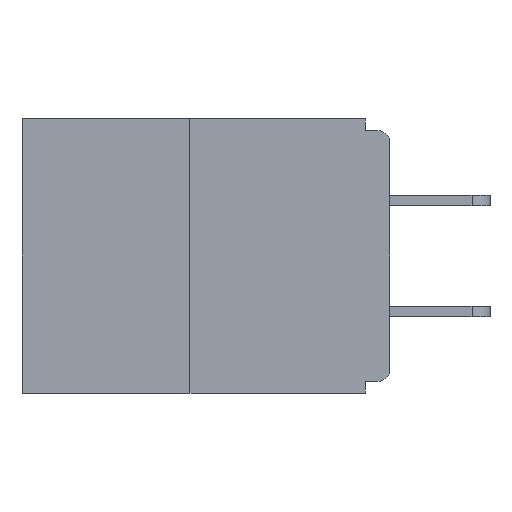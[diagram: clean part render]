
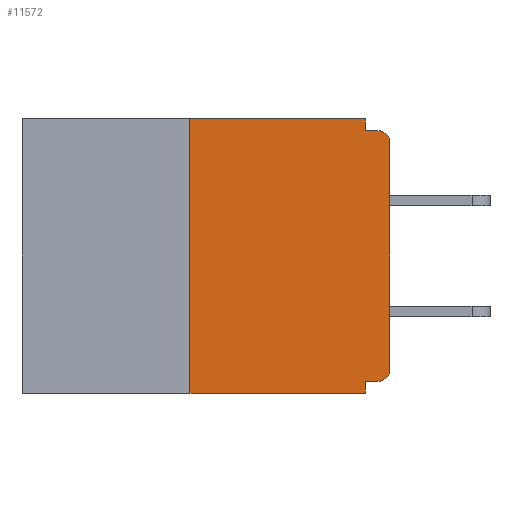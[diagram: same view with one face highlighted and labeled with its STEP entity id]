
A CAD part, left-side view. The second image highlights one B-rep face of the part: STEP entity #11572.
In plain terms, the highlighted planar face has unit normal (-1, 0, 0).
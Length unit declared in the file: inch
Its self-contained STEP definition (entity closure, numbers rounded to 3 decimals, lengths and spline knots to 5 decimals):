
#219 = DIRECTION ( 'NONE',  ( 0., -1., 0. ) ) ;
#304 = EDGE_CURVE ( 'NONE', #12619, #564, #17571, .T. ) ;
#513 = ORIENTED_EDGE ( 'NONE', *, *, #15176, .F. ) ;
#564 = VERTEX_POINT ( 'NONE', #8336 ) ;
#835 = DIRECTION ( 'NONE',  ( -1., 0., 0. ) ) ;
#873 = CARTESIAN_POINT ( 'NONE',  ( 0., 0.015, -0.313 ) ) ;
#932 = DIRECTION ( 'NONE',  ( 0., 1., 0. ) ) ;
#1701 = CARTESIAN_POINT ( 'NONE',  ( 0., 0.031, 0. ) ) ;
#1729 = EDGE_CURVE ( 'NONE', #12619, #13529, #4826, .T. ) ;
#1971 = ORIENTED_EDGE ( 'NONE', *, *, #9385, .F. ) ;
#2125 = ORIENTED_EDGE ( 'NONE', *, *, #1729, .F. ) ;
#2174 = CARTESIAN_POINT ( 'NONE',  ( 0., 0.015, -0.03 ) ) ;
#2514 = EDGE_CURVE ( 'NONE', #12037, #9377, #8472, .T. ) ;
#2839 = VECTOR ( 'NONE', #4182, 39.37008 ) ;
#2876 = DIRECTION ( 'NONE',  ( 0., 0., -1. ) ) ;
#3122 = CARTESIAN_POINT ( 'NONE',  ( 0., 0.25, -0.343 ) ) ;
#3673 = ORIENTED_EDGE ( 'NONE', *, *, #17015, .T. ) ;
#3957 = VERTEX_POINT ( 'NONE', #3960 ) ;
#3960 = CARTESIAN_POINT ( 'NONE',  ( 0., 0., -0.03 ) ) ;
#4057 = CARTESIAN_POINT ( 'NONE',  ( 0., 0., 0. ) ) ;
#4182 = DIRECTION ( 'NONE',  ( 0., 0., 1. ) ) ;
#4380 = CARTESIAN_POINT ( 'NONE',  ( 0., 0.031, 0. ) ) ;
#4469 = ORIENTED_EDGE ( 'NONE', *, *, #5813, .F. ) ;
#4684 = ORIENTED_EDGE ( 'NONE', *, *, #2514, .F. ) ;
#4826 = LINE ( 'NONE', #6350, #11333 ) ;
#4979 = DIRECTION ( 'NONE',  ( 1., 0., 0. ) ) ;
#5468 = EDGE_CURVE ( 'NONE', #15251, #14833, #17730, .T. ) ;
#5727 = CARTESIAN_POINT ( 'NONE',  ( 0., 0.031, -0.015 ) ) ;
#5813 = EDGE_CURVE ( 'NONE', #13546, #564, #14965, .T. ) ;
#6093 = ORIENTED_EDGE ( 'NONE', *, *, #8663, .T. ) ;
#6254 = CARTESIAN_POINT ( 'NONE',  ( 0., 0., -0.015 ) ) ;
#6350 = CARTESIAN_POINT ( 'NONE',  ( 0., 0.25, 0. ) ) ;
#6360 = DIRECTION ( 'NONE',  ( 0., 0., -1. ) ) ;
#6596 = EDGE_LOOP ( 'NONE', ( #1971, #2125, #8793, #4469, #10486, #12529, #6093, #3673, #513, #4684 ) ) ;
#6995 = CARTESIAN_POINT ( 'NONE',  ( 0., 0.46, 0. ) ) ;
#7605 = CARTESIAN_POINT ( 'NONE',  ( 0., 0.25, 0. ) ) ;
#7823 = VECTOR ( 'NONE', #2876, 39.37008 ) ;
#7994 = LINE ( 'NONE', #4057, #2839 ) ;
#8002 = CARTESIAN_POINT ( 'NONE',  ( 0., 0.015, -0.015 ) ) ;
#8170 = VECTOR ( 'NONE', #219, 39.37008 ) ;
#8336 = CARTESIAN_POINT ( 'NONE',  ( 0., 0.031, -0.343 ) ) ;
#8472 = LINE ( 'NONE', #4380, #7823 ) ;
#8663 = EDGE_CURVE ( 'NONE', #14833, #3957, #7994, .T. ) ;
#8750 = CARTESIAN_POINT ( 'NONE',  ( 0., 0.46, -0.343 ) ) ;
#8793 = ORIENTED_EDGE ( 'NONE', *, *, #304, .T. ) ;
#9377 = VERTEX_POINT ( 'NONE', #5727 ) ;
#9385 = EDGE_CURVE ( 'NONE', #13529, #12037, #9483, .T. ) ;
#9483 = LINE ( 'NONE', #6995, #8170 ) ;
#9524 = CARTESIAN_POINT ( 'NONE',  ( 0., 0.015, -0.328 ) ) ;
#9771 = VECTOR ( 'NONE', #932, 39.37008 ) ;
#10486 = ORIENTED_EDGE ( 'NONE', *, *, #17710, .F. ) ;
#10730 = VECTOR ( 'NONE', #12726, 39.37008 ) ;
#11303 = LINE ( 'NONE', #13405, #9771 ) ;
#11333 = VECTOR ( 'NONE', #13299, 39.37008 ) ;
#11572 = ADVANCED_FACE ( 'NONE', ( #11594 ), #11887, .F. ) ;
#11594 = FACE_OUTER_BOUND ( 'NONE', #6596, .T. ) ;
#11887 = PLANE ( 'NONE',  #15050 ) ;
#12037 = VERTEX_POINT ( 'NONE', #1701 ) ;
#12080 = CARTESIAN_POINT ( 'NONE',  ( 0., 0., -0.313 ) ) ;
#12313 = VECTOR ( 'NONE', #14743, 39.37008 ) ;
#12529 = ORIENTED_EDGE ( 'NONE', *, *, #5468, .T. ) ;
#12619 = VERTEX_POINT ( 'NONE', #3122 ) ;
#12726 = DIRECTION ( 'NONE',  ( 0., -1., 0. ) ) ;
#13048 = DIRECTION ( 'NONE',  ( -1., 0., 0. ) ) ;
#13299 = DIRECTION ( 'NONE',  ( 0., 0., 1. ) ) ;
#13405 = CARTESIAN_POINT ( 'NONE',  ( 0., 0., -0.328 ) ) ;
#13502 = VERTEX_POINT ( 'NONE', #8002 ) ;
#13529 = VERTEX_POINT ( 'NONE', #7605 ) ;
#13546 = VERTEX_POINT ( 'NONE', #17337 ) ;
#13964 = DIRECTION ( 'NONE',  ( 0., 0., -1. ) ) ;
#14298 = VECTOR ( 'NONE', #13964, 39.37008 ) ;
#14330 = DIRECTION ( 'NONE',  ( 0., 0., -1. ) ) ;
#14651 = CARTESIAN_POINT ( 'NONE',  ( 0., 0.46, 0. ) ) ;
#14743 = DIRECTION ( 'NONE',  ( 0., -1., 0. ) ) ;
#14833 = VERTEX_POINT ( 'NONE', #12080 ) ;
#14965 = LINE ( 'NONE', #15049, #14298 ) ;
#15002 = AXIS2_PLACEMENT_3D ( 'NONE', #2174, #835, #15651 ) ;
#15049 = CARTESIAN_POINT ( 'NONE',  ( 0., 0.031, -0.343 ) ) ;
#15050 = AXIS2_PLACEMENT_3D ( 'NONE', #14651, #4979, #6360 ) ;
#15176 = EDGE_CURVE ( 'NONE', #9377, #13502, #17236, .T. ) ;
#15251 = VERTEX_POINT ( 'NONE', #9524 ) ;
#15397 = CIRCLE ( 'NONE', #15002, 0.015 ) ;
#15651 = DIRECTION ( 'NONE',  ( 0., 0., -1. ) ) ;
#16132 = AXIS2_PLACEMENT_3D ( 'NONE', #873, #13048, #14330 ) ;
#17015 = EDGE_CURVE ( 'NONE', #3957, #13502, #15397, .T. ) ;
#17236 = LINE ( 'NONE', #6254, #12313 ) ;
#17337 = CARTESIAN_POINT ( 'NONE',  ( 0., 0.031, -0.328 ) ) ;
#17571 = LINE ( 'NONE', #8750, #10730 ) ;
#17710 = EDGE_CURVE ( 'NONE', #15251, #13546, #11303, .T. ) ;
#17730 = CIRCLE ( 'NONE', #16132, 0.015 ) ;
